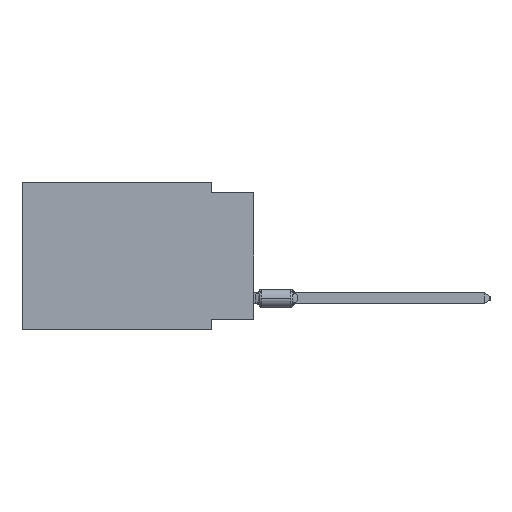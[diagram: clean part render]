
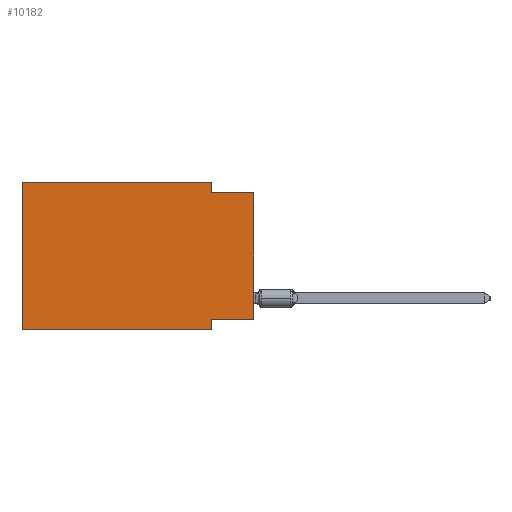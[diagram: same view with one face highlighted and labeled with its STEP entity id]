
A CAD part, left-side view. The second image highlights one B-rep face of the part: STEP entity #10182.
In plain terms, the highlighted planar face has unit normal (-1, 0, 0).
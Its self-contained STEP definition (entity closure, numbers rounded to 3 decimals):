
#398 = ORIENTED_EDGE ( 'NONE', *, *, #25950, .F. ) ;
#442 = VECTOR ( 'NONE', #62530, 1000. ) ;
#2294 = VECTOR ( 'NONE', #8161, 1000. ) ;
#7831 = CARTESIAN_POINT ( 'NONE',  ( 0., 13.97, 0. ) ) ;
#8161 = DIRECTION ( 'NONE',  ( 0., 0., 1. ) ) ;
#8508 = EDGE_CURVE ( 'NONE', #35248, #51303, #22802, .T. ) ;
#10030 = ORIENTED_EDGE ( 'NONE', *, *, #53096, .F. ) ;
#10182 = ADVANCED_FACE ( 'NONE', ( #17926 ), #18266, .F. ) ;
#10525 = CARTESIAN_POINT ( 'NONE',  ( 0., 2.54, -0.635 ) ) ;
#11531 = CARTESIAN_POINT ( 'NONE',  ( 0., 0., 0. ) ) ;
#11843 = CARTESIAN_POINT ( 'NONE',  ( 0., 13.97, 0. ) ) ;
#13139 = DIRECTION ( 'NONE',  ( 0., 0., -1. ) ) ;
#14192 = CARTESIAN_POINT ( 'NONE',  ( 0., 2.54, -8.89 ) ) ;
#14398 = ORIENTED_EDGE ( 'NONE', *, *, #18481, .T. ) ;
#14731 = DIRECTION ( 'NONE',  ( 0., -1., 0. ) ) ;
#15074 = LINE ( 'NONE', #31171, #53026 ) ;
#15770 = VERTEX_POINT ( 'NONE', #42006 ) ;
#16972 = DIRECTION ( 'NONE',  ( 0., -1., 0. ) ) ;
#17418 = CARTESIAN_POINT ( 'NONE',  ( 0., 13.97, 0. ) ) ;
#17526 = VECTOR ( 'NONE', #16972, 1000. ) ;
#17926 = FACE_OUTER_BOUND ( 'NONE', #44204, .T. ) ;
#18266 = PLANE ( 'NONE',  #40896 ) ;
#18481 = EDGE_CURVE ( 'NONE', #61376, #35572, #15074, .T. ) ;
#18757 = VERTEX_POINT ( 'NONE', #7831 ) ;
#20117 = CARTESIAN_POINT ( 'NONE',  ( 0., 2.54, 0. ) ) ;
#22802 = LINE ( 'NONE', #63970, #17526 ) ;
#22927 = DIRECTION ( 'NONE',  ( 0., 1., 0. ) ) ;
#24317 = CARTESIAN_POINT ( 'NONE',  ( 0., 0., -8.255 ) ) ;
#25006 = ORIENTED_EDGE ( 'NONE', *, *, #31790, .F. ) ;
#25950 = EDGE_CURVE ( 'NONE', #61376, #18757, #32873, .T. ) ;
#26629 = VERTEX_POINT ( 'NONE', #24317 ) ;
#29932 = ORIENTED_EDGE ( 'NONE', *, *, #8508, .F. ) ;
#30649 = LINE ( 'NONE', #14192, #442 ) ;
#31171 = CARTESIAN_POINT ( 'NONE',  ( 0., 13.97, -8.89 ) ) ;
#31790 = EDGE_CURVE ( 'NONE', #52831, #35248, #55138, .T. ) ;
#32742 = CARTESIAN_POINT ( 'NONE',  ( 0., 0., -0.635 ) ) ;
#32873 = LINE ( 'NONE', #17418, #2294 ) ;
#33223 = LINE ( 'NONE', #59976, #67585 ) ;
#33428 = DIRECTION ( 'NONE',  ( 0., -1., 0. ) ) ;
#33812 = EDGE_CURVE ( 'NONE', #18757, #52831, #48896, .T. ) ;
#35248 = VERTEX_POINT ( 'NONE', #10525 ) ;
#35572 = VERTEX_POINT ( 'NONE', #56446 ) ;
#37150 = VECTOR ( 'NONE', #41054, 1000. ) ;
#37936 = DIRECTION ( 'NONE',  ( 0., 0., 1. ) ) ;
#38859 = DIRECTION ( 'NONE',  ( 1., 0., 0. ) ) ;
#40896 = AXIS2_PLACEMENT_3D ( 'NONE', #49186, #38859, #13139 ) ;
#41054 = DIRECTION ( 'NONE',  ( 0., 0., -1. ) ) ;
#42006 = CARTESIAN_POINT ( 'NONE',  ( 0., 2.54, -8.255 ) ) ;
#43431 = LINE ( 'NONE', #11531, #54531 ) ;
#44019 = EDGE_CURVE ( 'NONE', #26629, #51303, #43431, .T. ) ;
#44204 = EDGE_LOOP ( 'NONE', ( #61517, #29932, #25006, #45277, #398, #14398, #59076, #10030 ) ) ;
#45277 = ORIENTED_EDGE ( 'NONE', *, *, #33812, .F. ) ;
#48896 = LINE ( 'NONE', #11843, #58200 ) ;
#49186 = CARTESIAN_POINT ( 'NONE',  ( 0., 13.97, 0. ) ) ;
#49305 = CARTESIAN_POINT ( 'NONE',  ( 0., 2.54, 0. ) ) ;
#51303 = VERTEX_POINT ( 'NONE', #32742 ) ;
#51511 = CARTESIAN_POINT ( 'NONE',  ( 0., 13.97, -8.89 ) ) ;
#52831 = VERTEX_POINT ( 'NONE', #49305 ) ;
#53026 = VECTOR ( 'NONE', #14731, 1000. ) ;
#53096 = EDGE_CURVE ( 'NONE', #26629, #15770, #33223, .T. ) ;
#54531 = VECTOR ( 'NONE', #37936, 1000. ) ;
#55138 = LINE ( 'NONE', #20117, #37150 ) ;
#56446 = CARTESIAN_POINT ( 'NONE',  ( 0., 2.54, -8.89 ) ) ;
#58200 = VECTOR ( 'NONE', #33428, 1000. ) ;
#59076 = ORIENTED_EDGE ( 'NONE', *, *, #62291, .F. ) ;
#59976 = CARTESIAN_POINT ( 'NONE',  ( 0., 0., -8.255 ) ) ;
#61376 = VERTEX_POINT ( 'NONE', #51511 ) ;
#61517 = ORIENTED_EDGE ( 'NONE', *, *, #44019, .T. ) ;
#62291 = EDGE_CURVE ( 'NONE', #15770, #35572, #30649, .T. ) ;
#62530 = DIRECTION ( 'NONE',  ( 0., 0., -1. ) ) ;
#63970 = CARTESIAN_POINT ( 'NONE',  ( 0., 0., -0.635 ) ) ;
#67585 = VECTOR ( 'NONE', #22927, 1000. ) ;
